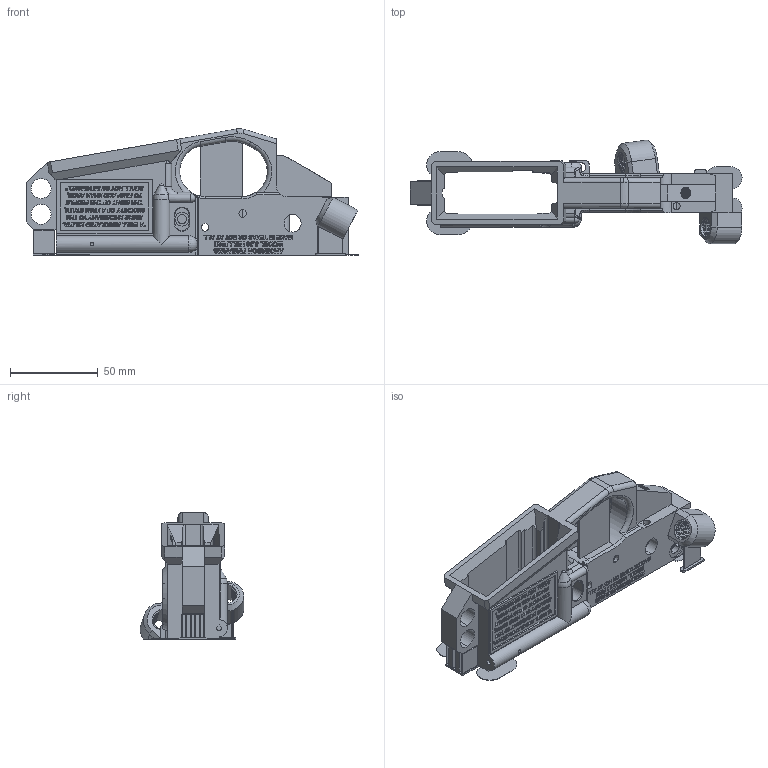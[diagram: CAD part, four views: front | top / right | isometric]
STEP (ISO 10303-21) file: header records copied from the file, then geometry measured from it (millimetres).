
FILE_DESCRIPTION (( 'STEP AP203' ), '1' );
FILE_NAME ('AF-HF-LR-PRT-001-STEP.STEP', '2020-12-04T13:04:14', ( '' ), ( '' ), 'SwSTEP 2.0', 'SolidWorks 2018', '' );
FILE_SCHEMA (( 'CONFIG_CONTROL_DESIGN' ));
Products named in the file (1): AF-HF-LR-PRT-001-STEP
Bounding box: 189.67 x 59.15 x 72.31 mm (x, y, z)
Volume: 102690.6 mm3; surface area: 75943.7 mm2
Topology: 5 solids, 5 shells, 3350 faces, 9167 edges, 6067 vertices
Faces by surface type: plane 2237, bspline 768, cylinder 300, torus 22, cone 19, sphere 4
Entity records: 186620 total; most frequent: CARTESIAN_POINT 107768, ORIENTED_EDGE 18322, DIRECTION 12890, EDGE_CURVE 9161, LINE 6710, VECTOR 6710, VERTEX_POINT 6066, EDGE_LOOP 3641
